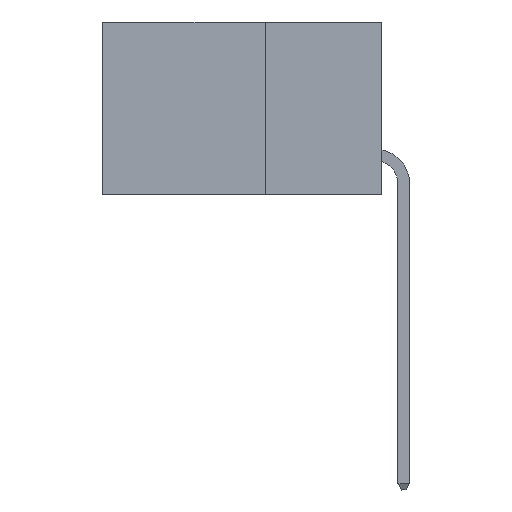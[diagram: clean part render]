
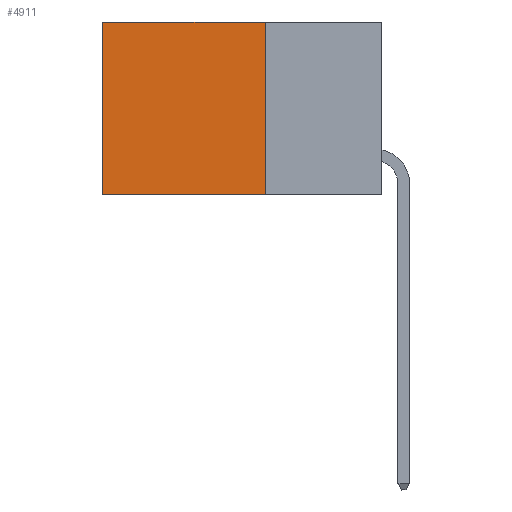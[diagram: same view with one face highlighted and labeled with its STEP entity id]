
A CAD part, left-side view. The second image highlights one B-rep face of the part: STEP entity #4911.
In plain terms, the highlighted planar face has unit normal (-1, 0, 0).
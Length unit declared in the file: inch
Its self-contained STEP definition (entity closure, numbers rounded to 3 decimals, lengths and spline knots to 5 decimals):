
#591 = ORIENTED_EDGE ( 'NONE', *, *, #7975, .F. ) ;
#718 = PLANE ( 'NONE',  #13404 ) ;
#914 = EDGE_CURVE ( 'NONE', #8136, #8000, #4198, .T. ) ;
#1609 = VECTOR ( 'NONE', #11332, 39.37008 ) ;
#1944 = VERTEX_POINT ( 'NONE', #14470 ) ;
#2773 = DIRECTION ( 'NONE',  ( 0., 0., -1. ) ) ;
#2831 = CARTESIAN_POINT ( 'NONE',  ( 0.2875, 0.25, 0. ) ) ;
#2995 = EDGE_CURVE ( 'NONE', #1944, #8136, #10223, .T. ) ;
#3411 = VECTOR ( 'NONE', #11661, 39.37008 ) ;
#3434 = DIRECTION ( 'NONE',  ( 0., 0., -1. ) ) ;
#3545 = ORIENTED_EDGE ( 'NONE', *, *, #11089, .F. ) ;
#4198 = LINE ( 'NONE', #12730, #3411 ) ;
#4695 = EDGE_LOOP ( 'NONE', ( #5601, #3545, #591, #10864 ) ) ;
#4911 = ADVANCED_FACE ( 'NONE', ( #13892 ), #718, .F. ) ;
#5601 = ORIENTED_EDGE ( 'NONE', *, *, #914, .T. ) ;
#5920 = DIRECTION ( 'NONE',  ( 1., 0., 0. ) ) ;
#5951 = CARTESIAN_POINT ( 'NONE',  ( 0.2875, 0.25, -0.37 ) ) ;
#6102 = LINE ( 'NONE', #2831, #13196 ) ;
#7542 = VECTOR ( 'NONE', #10140, 39.37008 ) ;
#7975 = EDGE_CURVE ( 'NONE', #1944, #14110, #6102, .T. ) ;
#8000 = VERTEX_POINT ( 'NONE', #14214 ) ;
#8136 = VERTEX_POINT ( 'NONE', #10606 ) ;
#9923 = CARTESIAN_POINT ( 'NONE',  ( 0.2875, 0.25, -0.37 ) ) ;
#9958 = LINE ( 'NONE', #5951, #7542 ) ;
#10140 = DIRECTION ( 'NONE',  ( 0., 1., 0. ) ) ;
#10223 = LINE ( 'NONE', #12556, #1609 ) ;
#10606 = CARTESIAN_POINT ( 'NONE',  ( 0.2875, 0.6, 0. ) ) ;
#10864 = ORIENTED_EDGE ( 'NONE', *, *, #2995, .T. ) ;
#11089 = EDGE_CURVE ( 'NONE', #14110, #8000, #9958, .T. ) ;
#11332 = DIRECTION ( 'NONE',  ( 0., 1., 0. ) ) ;
#11661 = DIRECTION ( 'NONE',  ( 0., 0., -1. ) ) ;
#11974 = CARTESIAN_POINT ( 'NONE',  ( 0.2875, 0.25, 0. ) ) ;
#12556 = CARTESIAN_POINT ( 'NONE',  ( 0.2875, 0.25, 0. ) ) ;
#12730 = CARTESIAN_POINT ( 'NONE',  ( 0.2875, 0.6, 0. ) ) ;
#13196 = VECTOR ( 'NONE', #2773, 39.37008 ) ;
#13404 = AXIS2_PLACEMENT_3D ( 'NONE', #11974, #5920, #3434 ) ;
#13892 = FACE_OUTER_BOUND ( 'NONE', #4695, .T. ) ;
#14110 = VERTEX_POINT ( 'NONE', #9923 ) ;
#14214 = CARTESIAN_POINT ( 'NONE',  ( 0.2875, 0.6, -0.37 ) ) ;
#14470 = CARTESIAN_POINT ( 'NONE',  ( 0.2875, 0.25, 0. ) ) ;
